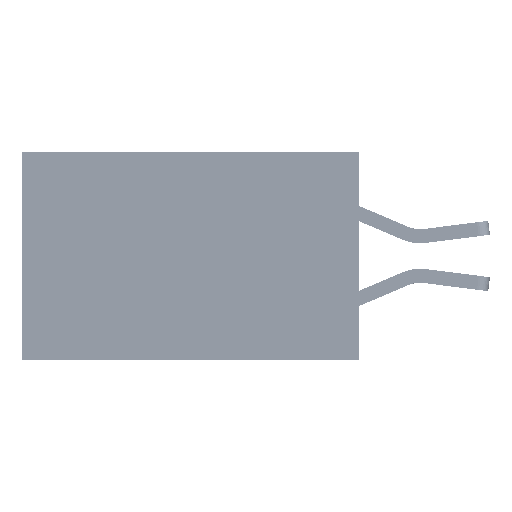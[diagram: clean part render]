
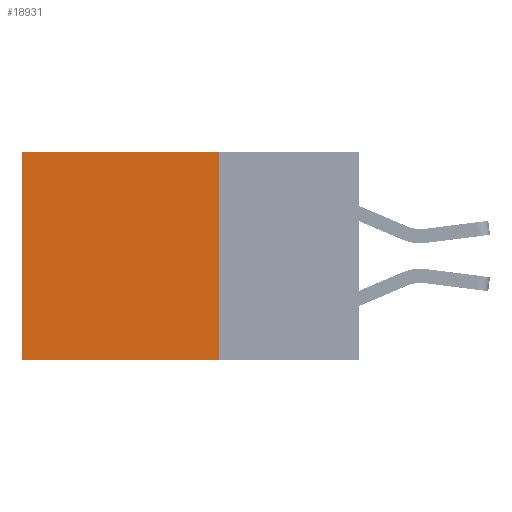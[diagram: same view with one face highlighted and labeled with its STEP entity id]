
A CAD part, left-side view. The second image highlights one B-rep face of the part: STEP entity #18931.
In plain terms, the highlighted planar face has unit normal (-1, 0, 0).
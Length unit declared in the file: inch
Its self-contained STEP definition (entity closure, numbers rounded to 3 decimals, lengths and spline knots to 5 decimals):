
#5107 = EDGE_CURVE ( 'NONE', #37519, #44777, #16864, .T. ) ;
#6262 = VECTOR ( 'NONE', #43484, 39.37008 ) ;
#7656 = CARTESIAN_POINT ( 'NONE',  ( 0.2875, 0.25, -0.37 ) ) ;
#8052 = ORIENTED_EDGE ( 'NONE', *, *, #5107, .F. ) ;
#13117 = DIRECTION ( 'NONE',  ( 0., 0., -1. ) ) ;
#14372 = ORIENTED_EDGE ( 'NONE', *, *, #41092, .F. ) ;
#14849 = FACE_OUTER_BOUND ( 'NONE', #49026, .T. ) ;
#15803 = VERTEX_POINT ( 'NONE', #41894 ) ;
#16864 = LINE ( 'NONE', #7656, #41071 ) ;
#17070 = ORIENTED_EDGE ( 'NONE', *, *, #30127, .T. ) ;
#17753 = DIRECTION ( 'NONE',  ( 0., 1., 0. ) ) ;
#18605 = CARTESIAN_POINT ( 'NONE',  ( 0.2875, 0.25, -0.37 ) ) ;
#18931 = ADVANCED_FACE ( 'NONE', ( #14849 ), #44566, .F. ) ;
#19306 = DIRECTION ( 'NONE',  ( 0., 1., 0. ) ) ;
#21876 = CARTESIAN_POINT ( 'NONE',  ( 0.2875, 0.25, 0. ) ) ;
#22697 = LINE ( 'NONE', #28310, #42732 ) ;
#23060 = VECTOR ( 'NONE', #17753, 39.37008 ) ;
#25201 = VERTEX_POINT ( 'NONE', #45878 ) ;
#26035 = AXIS2_PLACEMENT_3D ( 'NONE', #21876, #29482, #30322 ) ;
#26510 = CARTESIAN_POINT ( 'NONE',  ( 0.2875, 0.6, -0.37 ) ) ;
#28310 = CARTESIAN_POINT ( 'NONE',  ( 0.2875, 0.25, 0. ) ) ;
#29222 = CARTESIAN_POINT ( 'NONE',  ( 0.2875, 0.25, 0. ) ) ;
#29482 = DIRECTION ( 'NONE',  ( 1., 0., 0. ) ) ;
#29704 = LINE ( 'NONE', #29222, #23060 ) ;
#30127 = EDGE_CURVE ( 'NONE', #15803, #25201, #29704, .T. ) ;
#30322 = DIRECTION ( 'NONE',  ( 0., 0., -1. ) ) ;
#31430 = ORIENTED_EDGE ( 'NONE', *, *, #42590, .T. ) ;
#32279 = CARTESIAN_POINT ( 'NONE',  ( 0.2875, 0.6, 0. ) ) ;
#37519 = VERTEX_POINT ( 'NONE', #18605 ) ;
#41071 = VECTOR ( 'NONE', #19306, 39.37008 ) ;
#41092 = EDGE_CURVE ( 'NONE', #15803, #37519, #22697, .T. ) ;
#41894 = CARTESIAN_POINT ( 'NONE',  ( 0.2875, 0.25, 0. ) ) ;
#42590 = EDGE_CURVE ( 'NONE', #25201, #44777, #43199, .T. ) ;
#42732 = VECTOR ( 'NONE', #13117, 39.37008 ) ;
#43199 = LINE ( 'NONE', #32279, #6262 ) ;
#43484 = DIRECTION ( 'NONE',  ( 0., 0., -1. ) ) ;
#44566 = PLANE ( 'NONE',  #26035 ) ;
#44777 = VERTEX_POINT ( 'NONE', #26510 ) ;
#45878 = CARTESIAN_POINT ( 'NONE',  ( 0.2875, 0.6, 0. ) ) ;
#49026 = EDGE_LOOP ( 'NONE', ( #31430, #8052, #14372, #17070 ) ) ;
